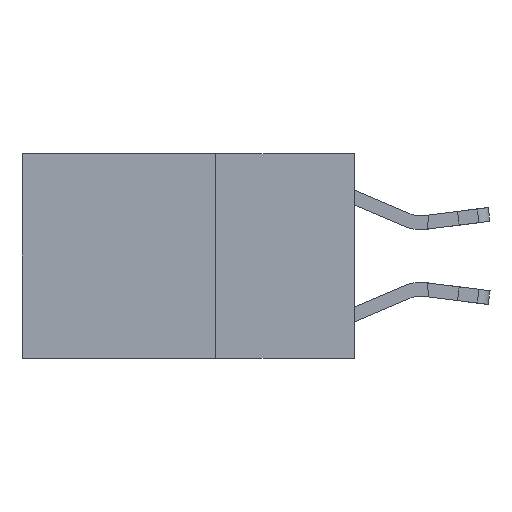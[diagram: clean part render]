
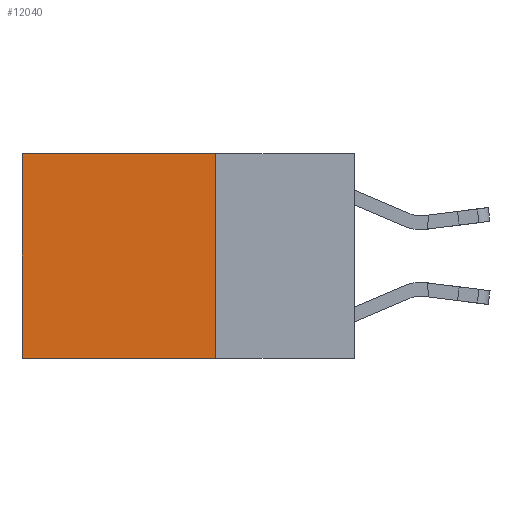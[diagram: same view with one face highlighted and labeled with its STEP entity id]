
A CAD part, left-side view. The second image highlights one B-rep face of the part: STEP entity #12040.
In plain terms, the highlighted planar face has unit normal (-1, 0, 0).
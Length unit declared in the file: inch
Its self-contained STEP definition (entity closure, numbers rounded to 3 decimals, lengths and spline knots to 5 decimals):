
#559 = VECTOR ( 'NONE', #19988, 39.37008 ) ;
#668 = DIRECTION ( 'NONE',  ( 0., 0., -1. ) ) ;
#849 = CARTESIAN_POINT ( 'NONE',  ( 0.2625, 0.25, -0.37 ) ) ;
#1913 = CARTESIAN_POINT ( 'NONE',  ( 0.2625, 0.6, 0. ) ) ;
#2337 = CARTESIAN_POINT ( 'NONE',  ( 0.2625, 0.25, 0. ) ) ;
#3450 = VECTOR ( 'NONE', #12844, 39.37008 ) ;
#4050 = LINE ( 'NONE', #10932, #3450 ) ;
#4130 = EDGE_CURVE ( 'NONE', #22882, #20488, #14060, .T. ) ;
#4410 = VERTEX_POINT ( 'NONE', #9343 ) ;
#5687 = AXIS2_PLACEMENT_3D ( 'NONE', #10260, #12171, #668 ) ;
#6260 = EDGE_CURVE ( 'NONE', #18241, #4410, #4050, .T. ) ;
#6957 = DIRECTION ( 'NONE',  ( 0., 1., 0. ) ) ;
#8092 = DIRECTION ( 'NONE',  ( 0., 1., 0. ) ) ;
#8593 = CARTESIAN_POINT ( 'NONE',  ( 0.2625, 0.25, 0. ) ) ;
#9343 = CARTESIAN_POINT ( 'NONE',  ( 0.2625, 0.6, -0.37 ) ) ;
#9412 = LINE ( 'NONE', #849, #24499 ) ;
#9926 = EDGE_CURVE ( 'NONE', #20488, #4410, #9412, .T. ) ;
#10260 = CARTESIAN_POINT ( 'NONE',  ( 0.2625, 0.25, 0. ) ) ;
#10932 = CARTESIAN_POINT ( 'NONE',  ( 0.2625, 0.6, 0. ) ) ;
#11141 = ORIENTED_EDGE ( 'NONE', *, *, #4130, .F. ) ;
#11639 = EDGE_LOOP ( 'NONE', ( #21420, #12574, #11141, #23871 ) ) ;
#12040 = ADVANCED_FACE ( 'NONE', ( #22347 ), #17573, .F. ) ;
#12171 = DIRECTION ( 'NONE',  ( 1., 0., 0. ) ) ;
#12574 = ORIENTED_EDGE ( 'NONE', *, *, #9926, .F. ) ;
#12844 = DIRECTION ( 'NONE',  ( 0., 0., -1. ) ) ;
#12855 = EDGE_CURVE ( 'NONE', #22882, #18241, #20283, .T. ) ;
#12902 = CARTESIAN_POINT ( 'NONE',  ( 0.2625, 0.25, -0.37 ) ) ;
#14060 = LINE ( 'NONE', #8593, #559 ) ;
#15232 = VECTOR ( 'NONE', #6957, 39.37008 ) ;
#17573 = PLANE ( 'NONE',  #5687 ) ;
#18241 = VERTEX_POINT ( 'NONE', #1913 ) ;
#19988 = DIRECTION ( 'NONE',  ( 0., 0., -1. ) ) ;
#20183 = CARTESIAN_POINT ( 'NONE',  ( 0.2625, 0.25, 0. ) ) ;
#20283 = LINE ( 'NONE', #20183, #15232 ) ;
#20488 = VERTEX_POINT ( 'NONE', #12902 ) ;
#21420 = ORIENTED_EDGE ( 'NONE', *, *, #6260, .T. ) ;
#22347 = FACE_OUTER_BOUND ( 'NONE', #11639, .T. ) ;
#22882 = VERTEX_POINT ( 'NONE', #2337 ) ;
#23871 = ORIENTED_EDGE ( 'NONE', *, *, #12855, .T. ) ;
#24499 = VECTOR ( 'NONE', #8092, 39.37008 ) ;
